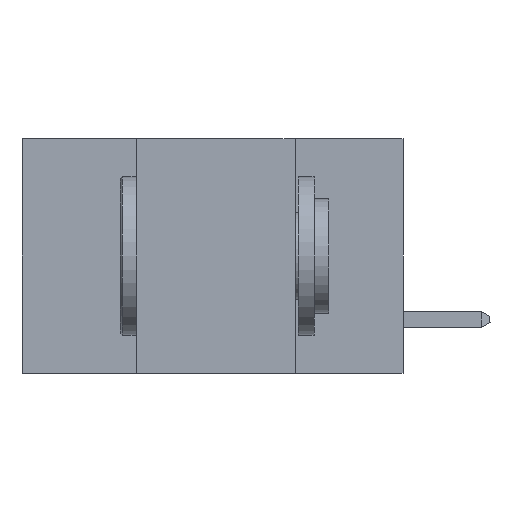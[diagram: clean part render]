
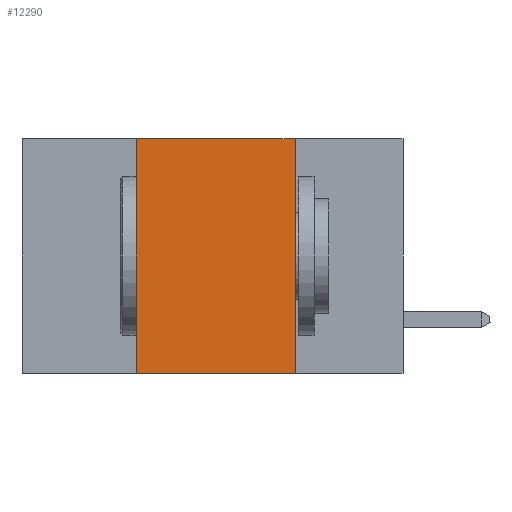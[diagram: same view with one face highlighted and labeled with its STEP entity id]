
A CAD part, left-side view. The second image highlights one B-rep face of the part: STEP entity #12290.
In plain terms, the highlighted planar face has unit normal (-1, 0, 0).
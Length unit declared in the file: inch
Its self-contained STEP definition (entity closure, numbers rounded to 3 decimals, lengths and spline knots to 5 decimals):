
#4 = CARTESIAN_POINT ( 'NONE',  ( 0., 0.17, -0.37 ) ) ;
#266 = ORIENTED_EDGE ( 'NONE', *, *, #16450, .F. ) ;
#529 = CARTESIAN_POINT ( 'NONE',  ( 0., 0.17, 0. ) ) ;
#1291 = CARTESIAN_POINT ( 'NONE',  ( 0., 0.42, 0. ) ) ;
#1549 = VECTOR ( 'NONE', #16271, 39.37008 ) ;
#2007 = LINE ( 'NONE', #17114, #1549 ) ;
#5526 = PLANE ( 'NONE',  #17765 ) ;
#5675 = VERTEX_POINT ( 'NONE', #1291 ) ;
#5715 = VERTEX_POINT ( 'NONE', #4 ) ;
#5839 = EDGE_CURVE ( 'NONE', #9617, #5715, #2007, .T. ) ;
#6492 = DIRECTION ( 'NONE',  ( 0., 0., -1. ) ) ;
#7014 = VECTOR ( 'NONE', #10778, 39.37008 ) ;
#7016 = DIRECTION ( 'NONE',  ( 1., 0., 0. ) ) ;
#7478 = EDGE_CURVE ( 'NONE', #9617, #5675, #15321, .T. ) ;
#8102 = CARTESIAN_POINT ( 'NONE',  ( 0., 0.6, 0. ) ) ;
#8347 = ORIENTED_EDGE ( 'NONE', *, *, #7478, .F. ) ;
#9617 = VERTEX_POINT ( 'NONE', #15860 ) ;
#9813 = FACE_OUTER_BOUND ( 'NONE', #11211, .T. ) ;
#10583 = CARTESIAN_POINT ( 'NONE',  ( 0., 0.42, 0. ) ) ;
#10778 = DIRECTION ( 'NONE',  ( 0., 0., 1. ) ) ;
#10860 = ORIENTED_EDGE ( 'NONE', *, *, #15855, .F. ) ;
#11211 = EDGE_LOOP ( 'NONE', ( #266, #10860, #8347, #13077 ) ) ;
#12290 = ADVANCED_FACE ( 'NONE', ( #9813 ), #5526, .F. ) ;
#12634 = VECTOR ( 'NONE', #6492, 39.37008 ) ;
#12930 = LINE ( 'NONE', #8102, #18691 ) ;
#13077 = ORIENTED_EDGE ( 'NONE', *, *, #5839, .T. ) ;
#15321 = LINE ( 'NONE', #10583, #7014 ) ;
#15841 = CARTESIAN_POINT ( 'NONE',  ( 0., 0.6, 0. ) ) ;
#15855 = EDGE_CURVE ( 'NONE', #5675, #18434, #12930, .T. ) ;
#15860 = CARTESIAN_POINT ( 'NONE',  ( 0., 0.42, -0.37 ) ) ;
#16271 = DIRECTION ( 'NONE',  ( 0., -1., 0. ) ) ;
#16450 = EDGE_CURVE ( 'NONE', #18434, #5715, #16512, .T. ) ;
#16512 = LINE ( 'NONE', #529, #12634 ) ;
#16833 = DIRECTION ( 'NONE',  ( 0., -1., 0. ) ) ;
#17114 = CARTESIAN_POINT ( 'NONE',  ( 0., 0.6, -0.37 ) ) ;
#17243 = DIRECTION ( 'NONE',  ( 0., 0., -1. ) ) ;
#17765 = AXIS2_PLACEMENT_3D ( 'NONE', #15841, #7016, #17243 ) ;
#18434 = VERTEX_POINT ( 'NONE', #18790 ) ;
#18691 = VECTOR ( 'NONE', #16833, 39.37008 ) ;
#18790 = CARTESIAN_POINT ( 'NONE',  ( 0., 0.17, 0. ) ) ;
